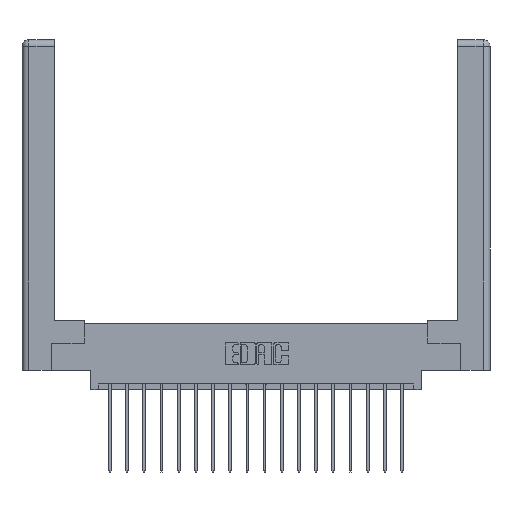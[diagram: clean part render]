
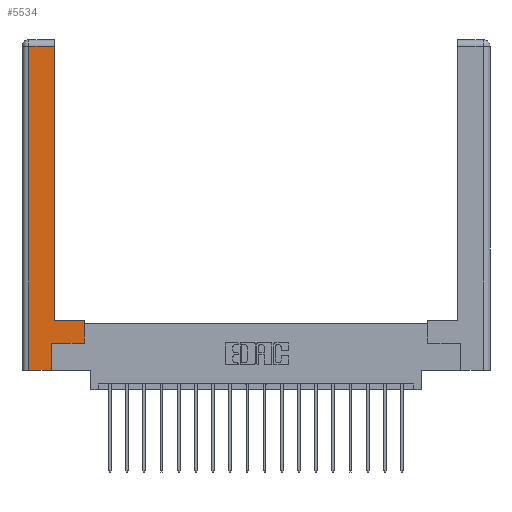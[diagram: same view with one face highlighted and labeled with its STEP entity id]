
A CAD part, top view. The second image highlights one B-rep face of the part: STEP entity #5534.
In plain terms, the highlighted planar face has unit normal (0, 0, 1).
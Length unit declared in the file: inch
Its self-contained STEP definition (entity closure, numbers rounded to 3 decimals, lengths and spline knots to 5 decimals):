
#417 = LINE ( 'NONE', #11114, #4990 ) ;
#632 = PLANE ( 'NONE',  #11072 ) ;
#779 = EDGE_CURVE ( 'NONE', #6958, #7471, #9205, .T. ) ;
#1398 = DIRECTION ( 'NONE',  ( 0., -1., 0. ) ) ;
#1670 = VECTOR ( 'NONE', #4258, 39.37008 ) ;
#1843 = ORIENTED_EDGE ( 'NONE', *, *, #8137, .T. ) ;
#2073 = VERTEX_POINT ( 'NONE', #7523 ) ;
#2114 = CARTESIAN_POINT ( 'NONE',  ( 0.265, 0., 0. ) ) ;
#2147 = CARTESIAN_POINT ( 'NONE',  ( 0.0615, 2.94, 0. ) ) ;
#2516 = EDGE_CURVE ( 'NONE', #5250, #2073, #18169, .T. ) ;
#2884 = CARTESIAN_POINT ( 'NONE',  ( 0.565, 0.45, 0. ) ) ;
#3114 = VERTEX_POINT ( 'NONE', #14301 ) ;
#3133 = EDGE_CURVE ( 'NONE', #2073, #6958, #417, .T. ) ;
#3657 = CARTESIAN_POINT ( 'NONE',  ( 0., 0., 0. ) ) ;
#4258 = DIRECTION ( 'NONE',  ( 0., 1., 0. ) ) ;
#4369 = VECTOR ( 'NONE', #1398, 39.37008 ) ;
#4990 = VECTOR ( 'NONE', #11248, 39.37008 ) ;
#5129 = DIRECTION ( 'NONE',  ( 0., 0., -1. ) ) ;
#5250 = VERTEX_POINT ( 'NONE', #12457 ) ;
#5534 = ADVANCED_FACE ( 'NONE', ( #11156 ), #632, .F. ) ;
#5614 = LINE ( 'NONE', #2114, #11851 ) ;
#5935 = CARTESIAN_POINT ( 'NONE',  ( 0.565, 0.245, 0. ) ) ;
#6029 = VECTOR ( 'NONE', #11983, 39.37008 ) ;
#6122 = EDGE_CURVE ( 'NONE', #7471, #19171, #5614, .T. ) ;
#6510 = LINE ( 'NONE', #5935, #6029 ) ;
#6958 = VERTEX_POINT ( 'NONE', #2147 ) ;
#6969 = VECTOR ( 'NONE', #13588, 39.37008 ) ;
#7039 = EDGE_CURVE ( 'NONE', #18488, #5250, #16610, .T. ) ;
#7435 = LINE ( 'NONE', #9502, #18161 ) ;
#7471 = VERTEX_POINT ( 'NONE', #11407 ) ;
#7521 = VERTEX_POINT ( 'NONE', #19586 ) ;
#7523 = CARTESIAN_POINT ( 'NONE',  ( 0.295, 2.94, 0. ) ) ;
#7604 = CARTESIAN_POINT ( 'NONE',  ( 0.265, 0., 0. ) ) ;
#8137 = EDGE_CURVE ( 'NONE', #7521, #3114, #6510, .T. ) ;
#8617 = CARTESIAN_POINT ( 'NONE',  ( 0.295, 3., 0. ) ) ;
#8655 = EDGE_CURVE ( 'NONE', #3114, #18488, #15101, .T. ) ;
#9205 = LINE ( 'NONE', #15265, #4369 ) ;
#9342 = EDGE_CURVE ( 'NONE', #19171, #7521, #7435, .T. ) ;
#9502 = CARTESIAN_POINT ( 'NONE',  ( 0.265, 0.245, 0. ) ) ;
#10403 = CARTESIAN_POINT ( 'NONE',  ( 0.295, 0.45, 0. ) ) ;
#10546 = ORIENTED_EDGE ( 'NONE', *, *, #9342, .T. ) ;
#10653 = VECTOR ( 'NONE', #12002, 39.37008 ) ;
#11072 = AXIS2_PLACEMENT_3D ( 'NONE', #3657, #5129, #19024 ) ;
#11114 = CARTESIAN_POINT ( 'NONE',  ( 0.0615, 2.94, 0. ) ) ;
#11156 = FACE_OUTER_BOUND ( 'NONE', #15930, .T. ) ;
#11248 = DIRECTION ( 'NONE',  ( -1., 0., 0. ) ) ;
#11407 = CARTESIAN_POINT ( 'NONE',  ( 0.0615, 0., 0. ) ) ;
#11851 = VECTOR ( 'NONE', #17299, 39.37008 ) ;
#11983 = DIRECTION ( 'NONE',  ( 1., 0., 0. ) ) ;
#12002 = DIRECTION ( 'NONE',  ( -1., 0., 0. ) ) ;
#12457 = CARTESIAN_POINT ( 'NONE',  ( 0.295, 0.45, 0. ) ) ;
#12562 = CARTESIAN_POINT ( 'NONE',  ( 0.565, 0.45, 0. ) ) ;
#12670 = ORIENTED_EDGE ( 'NONE', *, *, #8655, .T. ) ;
#13588 = DIRECTION ( 'NONE',  ( 0., 1., 0. ) ) ;
#14301 = CARTESIAN_POINT ( 'NONE',  ( 0.565, 0.245, 0. ) ) ;
#15101 = LINE ( 'NONE', #2884, #6969 ) ;
#15265 = CARTESIAN_POINT ( 'NONE',  ( 0.0615, 0., 0. ) ) ;
#15422 = ORIENTED_EDGE ( 'NONE', *, *, #2516, .T. ) ;
#15689 = DIRECTION ( 'NONE',  ( 0., 1., 0. ) ) ;
#15930 = EDGE_LOOP ( 'NONE', ( #15422, #17598, #16584, #16371, #10546, #1843, #12670, #16035 ) ) ;
#16035 = ORIENTED_EDGE ( 'NONE', *, *, #7039, .T. ) ;
#16371 = ORIENTED_EDGE ( 'NONE', *, *, #6122, .T. ) ;
#16584 = ORIENTED_EDGE ( 'NONE', *, *, #779, .T. ) ;
#16610 = LINE ( 'NONE', #10403, #10653 ) ;
#17299 = DIRECTION ( 'NONE',  ( 1., 0., 0. ) ) ;
#17598 = ORIENTED_EDGE ( 'NONE', *, *, #3133, .T. ) ;
#18161 = VECTOR ( 'NONE', #15689, 39.37008 ) ;
#18169 = LINE ( 'NONE', #8617, #1670 ) ;
#18488 = VERTEX_POINT ( 'NONE', #12562 ) ;
#19024 = DIRECTION ( 'NONE',  ( -1., 0., 0. ) ) ;
#19171 = VERTEX_POINT ( 'NONE', #7604 ) ;
#19586 = CARTESIAN_POINT ( 'NONE',  ( 0.265, 0.245, 0. ) ) ;
